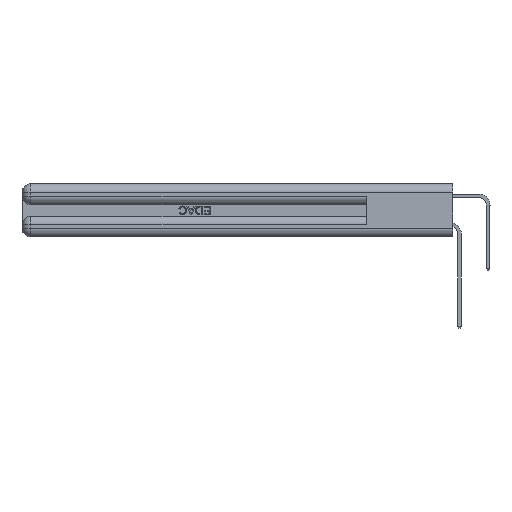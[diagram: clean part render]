
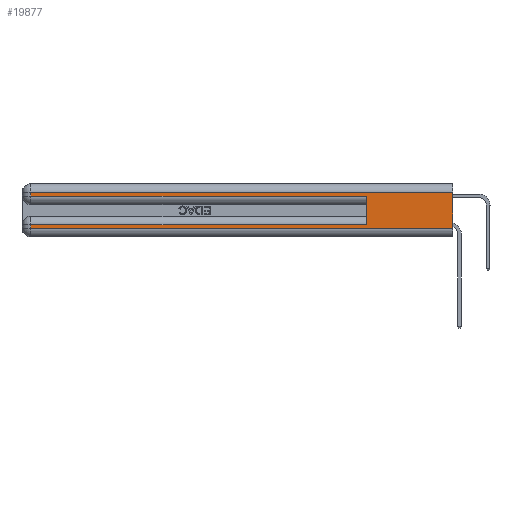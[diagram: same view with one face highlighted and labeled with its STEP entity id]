
A CAD part, left-side view. The second image highlights one B-rep face of the part: STEP entity #19877.
In plain terms, the highlighted planar face has unit normal (-1, 0, 0).
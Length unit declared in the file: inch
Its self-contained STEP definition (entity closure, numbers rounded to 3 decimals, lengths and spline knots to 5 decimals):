
#305 = FACE_OUTER_BOUND ( 'NONE', #45193, .T. ) ;
#1026 = VECTOR ( 'NONE', #16184, 39.37008 ) ;
#2066 = ORIENTED_EDGE ( 'NONE', *, *, #39692, .F. ) ;
#2241 = DIRECTION ( 'NONE',  ( 0., 0., -1. ) ) ;
#2432 = VECTOR ( 'NONE', #18785, 39.37008 ) ;
#3328 = EDGE_CURVE ( 'NONE', #39482, #19997, #12176, .T. ) ;
#3940 = CARTESIAN_POINT ( 'NONE',  ( 0., 0., 0.37 ) ) ;
#5166 = CARTESIAN_POINT ( 'NONE',  ( 0., 0.6, 0.145 ) ) ;
#6356 = EDGE_CURVE ( 'NONE', #19757, #26592, #6817, .T. ) ;
#6817 = LINE ( 'NONE', #27987, #13063 ) ;
#6908 = EDGE_CURVE ( 'NONE', #44757, #34102, #10774, .T. ) ;
#7665 = CARTESIAN_POINT ( 'NONE',  ( 0., 2.94, 0.37 ) ) ;
#7670 = DIRECTION ( 'NONE',  ( 1., 0., 0. ) ) ;
#7814 = DIRECTION ( 'NONE',  ( 0., 0., -1. ) ) ;
#9232 = LINE ( 'NONE', #10782, #46598 ) ;
#9840 = LINE ( 'NONE', #38603, #36510 ) ;
#10516 = ORIENTED_EDGE ( 'NONE', *, *, #6908, .T. ) ;
#10774 = LINE ( 'NONE', #12512, #1026 ) ;
#10782 = CARTESIAN_POINT ( 'NONE',  ( 0., 0., 0.31 ) ) ;
#11281 = CARTESIAN_POINT ( 'NONE',  ( 0., 2.94, 0.31 ) ) ;
#11570 = EDGE_CURVE ( 'NONE', #44376, #39482, #9232, .T. ) ;
#11913 = DIRECTION ( 'NONE',  ( 0., -1., 0. ) ) ;
#12068 = EDGE_CURVE ( 'NONE', #44376, #34102, #9840, .T. ) ;
#12088 = CARTESIAN_POINT ( 'NONE',  ( 0., 2.94, 0.37 ) ) ;
#12176 = LINE ( 'NONE', #12088, #2432 ) ;
#12318 = AXIS2_PLACEMENT_3D ( 'NONE', #3940, #7670, #33076 ) ;
#12512 = CARTESIAN_POINT ( 'NONE',  ( 0., 0., 0.06 ) ) ;
#12883 = CARTESIAN_POINT ( 'NONE',  ( 0., 2.94, 0.285 ) ) ;
#13063 = VECTOR ( 'NONE', #20682, 39.37008 ) ;
#14310 = VECTOR ( 'NONE', #45096, 39.37008 ) ;
#16184 = DIRECTION ( 'NONE',  ( 0., -1., 0. ) ) ;
#16674 = VERTEX_POINT ( 'NONE', #34170 ) ;
#18643 = CARTESIAN_POINT ( 'NONE',  ( 0., 0., 0.31 ) ) ;
#18785 = DIRECTION ( 'NONE',  ( 0., 0., -1. ) ) ;
#19179 = ORIENTED_EDGE ( 'NONE', *, *, #6356, .T. ) ;
#19757 = VERTEX_POINT ( 'NONE', #32464 ) ;
#19877 = ADVANCED_FACE ( 'NONE', ( #305 ), #22111, .F. ) ;
#19997 = VERTEX_POINT ( 'NONE', #12883 ) ;
#20036 = LINE ( 'NONE', #7665, #38138 ) ;
#20682 = DIRECTION ( 'NONE',  ( 0., 1., 0. ) ) ;
#22111 = PLANE ( 'NONE',  #12318 ) ;
#22448 = CARTESIAN_POINT ( 'NONE',  ( 0., 2.94, 0.06 ) ) ;
#23995 = LINE ( 'NONE', #5166, #14310 ) ;
#24216 = CARTESIAN_POINT ( 'NONE',  ( 0., 2.94, 0.085 ) ) ;
#24418 = ORIENTED_EDGE ( 'NONE', *, *, #3328, .T. ) ;
#26592 = VERTEX_POINT ( 'NONE', #24216 ) ;
#27987 = CARTESIAN_POINT ( 'NONE',  ( 0., 0., 0.085 ) ) ;
#28985 = ORIENTED_EDGE ( 'NONE', *, *, #12068, .F. ) ;
#31543 = LINE ( 'NONE', #37263, #39951 ) ;
#32432 = ORIENTED_EDGE ( 'NONE', *, *, #11570, .T. ) ;
#32464 = CARTESIAN_POINT ( 'NONE',  ( 0., 0.6, 0.085 ) ) ;
#33076 = DIRECTION ( 'NONE',  ( 0., 0., -1. ) ) ;
#34102 = VERTEX_POINT ( 'NONE', #44022 ) ;
#34170 = CARTESIAN_POINT ( 'NONE',  ( 0., 0.6, 0.285 ) ) ;
#34180 = EDGE_CURVE ( 'NONE', #19997, #16674, #31543, .T. ) ;
#35567 = ORIENTED_EDGE ( 'NONE', *, *, #44380, .T. ) ;
#36510 = VECTOR ( 'NONE', #2241, 39.37008 ) ;
#37263 = CARTESIAN_POINT ( 'NONE',  ( 0., 0., 0.285 ) ) ;
#37459 = ORIENTED_EDGE ( 'NONE', *, *, #34180, .T. ) ;
#38138 = VECTOR ( 'NONE', #7814, 39.37008 ) ;
#38603 = CARTESIAN_POINT ( 'NONE',  ( 0., 0., 0.37 ) ) ;
#39482 = VERTEX_POINT ( 'NONE', #11281 ) ;
#39692 = EDGE_CURVE ( 'NONE', #19757, #16674, #23995, .T. ) ;
#39729 = DIRECTION ( 'NONE',  ( 0., 1., 0. ) ) ;
#39951 = VECTOR ( 'NONE', #11913, 39.37008 ) ;
#44022 = CARTESIAN_POINT ( 'NONE',  ( 0., 0., 0.06 ) ) ;
#44376 = VERTEX_POINT ( 'NONE', #18643 ) ;
#44380 = EDGE_CURVE ( 'NONE', #26592, #44757, #20036, .T. ) ;
#44757 = VERTEX_POINT ( 'NONE', #22448 ) ;
#45096 = DIRECTION ( 'NONE',  ( 0., 0., 1. ) ) ;
#45193 = EDGE_LOOP ( 'NONE', ( #28985, #32432, #24418, #37459, #2066, #19179, #35567, #10516 ) ) ;
#46598 = VECTOR ( 'NONE', #39729, 39.37008 ) ;
